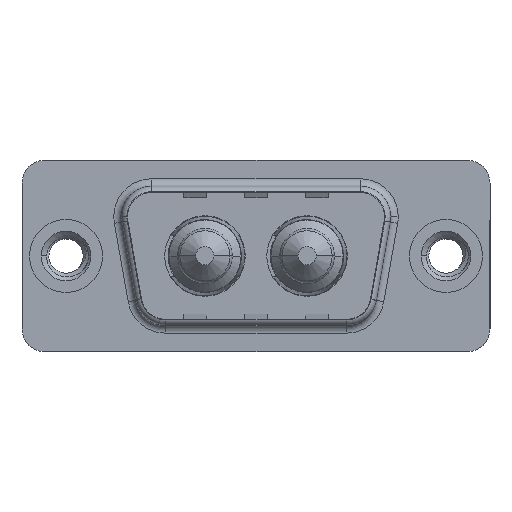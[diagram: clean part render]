
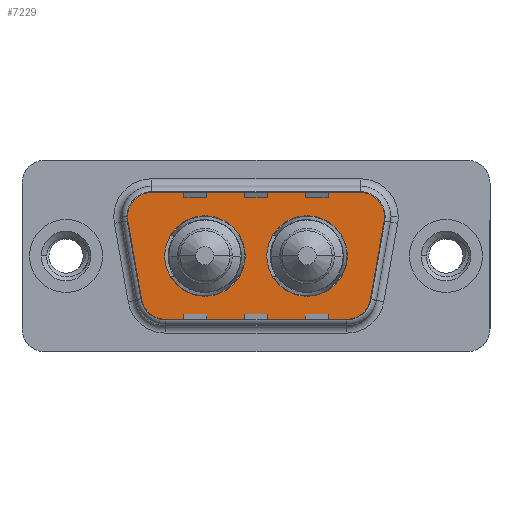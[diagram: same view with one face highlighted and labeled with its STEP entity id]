
A CAD part, top view. The second image highlights one B-rep face of the part: STEP entity #7229.
In plain terms, the highlighted planar face has unit normal (0, 0, 1).
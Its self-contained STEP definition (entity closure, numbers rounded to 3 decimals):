
#38 = VECTOR ( 'NONE', #4921, 1000. ) ;
#371 = CIRCLE ( 'NONE', #11608, 2.65 ) ;
#420 = DIRECTION ( 'NONE',  ( 0.174, -0.985, 0. ) ) ;
#428 = CARTESIAN_POINT ( 'NONE',  ( 19.564, 2.9, 0. ) ) ;
#515 = CIRCLE ( 'NONE', #10790, 2. ) ;
#672 = LINE ( 'NONE', #2986, #10633 ) ;
#941 = CARTESIAN_POINT ( 'NONE',  ( 18.51, 0., 0. ) ) ;
#1047 = DIRECTION ( 'NONE',  ( 0., 0., 1. ) ) ;
#1090 = VERTEX_POINT ( 'NONE', #8661 ) ;
#1092 = AXIS2_PLACEMENT_3D ( 'NONE', #3979, #5673, #10266 ) ;
#1099 = DIRECTION ( 'NONE',  ( -1., 0., 0. ) ) ;
#1525 = VERTEX_POINT ( 'NONE', #3818 ) ;
#1540 = VERTEX_POINT ( 'NONE', #10350 ) ;
#1951 = VERTEX_POINT ( 'NONE', #10084 ) ;
#2005 = CIRCLE ( 'NONE', #5672, 2.65 ) ;
#2106 = DIRECTION ( 'NONE',  ( 1., 0., 0. ) ) ;
#2252 = ORIENTED_EDGE ( 'NONE', *, *, #3138, .T. ) ;
#2335 = EDGE_CURVE ( 'NONE', #10232, #10680, #515, .T. ) ;
#2397 = DIRECTION ( 'NONE',  ( -1., 0., 0. ) ) ;
#2450 = CARTESIAN_POINT ( 'NONE',  ( 18.541, -2.9, 0. ) ) ;
#2498 = ORIENTED_EDGE ( 'NONE', *, *, #2335, .T. ) ;
#2545 = LINE ( 'NONE', #12049, #38 ) ;
#2569 = DIRECTION ( 'NONE',  ( 0., 0., 1. ) ) ;
#2676 = DIRECTION ( 'NONE',  ( 0., 0., 1. ) ) ;
#2828 = ORIENTED_EDGE ( 'NONE', *, *, #12010, .T. ) ;
#2935 = AXIS2_PLACEMENT_3D ( 'NONE', #4379, #2569, #2397 ) ;
#2966 = EDGE_CURVE ( 'NONE', #4654, #9092, #6804, .T. ) ;
#2982 = CARTESIAN_POINT ( 'NONE',  ( 6.459, -4.9, 0. ) ) ;
#2986 = CARTESIAN_POINT ( 'NONE',  ( 5.436, 4.9, 0. ) ) ;
#3026 = LINE ( 'NONE', #6037, #7998 ) ;
#3073 = EDGE_CURVE ( 'NONE', #3878, #1540, #5661, .T. ) ;
#3138 = EDGE_CURVE ( 'NONE', #9092, #10232, #2545, .T. ) ;
#3209 = EDGE_CURVE ( 'NONE', #1951, #8520, #6948, .T. ) ;
#3243 = DIRECTION ( 'NONE',  ( 1., 0., 0. ) ) ;
#3254 = CARTESIAN_POINT ( 'NONE',  ( 18.541, -4.9, 0. ) ) ;
#3329 = CARTESIAN_POINT ( 'NONE',  ( 15.86, 0., 0. ) ) ;
#3336 = DIRECTION ( 'NONE',  ( 1., 0., 0. ) ) ;
#3339 = CARTESIAN_POINT ( 'NONE',  ( 6.459, -2.9, 0. ) ) ;
#3362 = FACE_BOUND ( 'NONE', #8753, .T. ) ;
#3375 = DIRECTION ( 'NONE',  ( 0., 0., 1. ) ) ;
#3466 = DIRECTION ( 'NONE',  ( 0., 0., 1. ) ) ;
#3469 = DIRECTION ( 'NONE',  ( -1., 0., 0. ) ) ;
#3543 = EDGE_CURVE ( 'NONE', #11735, #9312, #10890, .T. ) ;
#3632 = PLANE ( 'NONE',  #6973 ) ;
#3774 = ORIENTED_EDGE ( 'NONE', *, *, #3543, .T. ) ;
#3778 = LINE ( 'NONE', #2982, #6375 ) ;
#3818 = CARTESIAN_POINT ( 'NONE',  ( 19.564, 4.9, 0. ) ) ;
#3878 = VERTEX_POINT ( 'NONE', #7794 ) ;
#3979 = CARTESIAN_POINT ( 'NONE',  ( 5.436, 2.9, 0. ) ) ;
#4060 = CARTESIAN_POINT ( 'NONE',  ( 18.541, -2.9, 0. ) ) ;
#4292 = DIRECTION ( 'NONE',  ( 1., 0., 0. ) ) ;
#4330 = CARTESIAN_POINT ( 'NONE',  ( 3.466, 2.553, 0. ) ) ;
#4379 = CARTESIAN_POINT ( 'NONE',  ( 19.564, 2.9, 0. ) ) ;
#4527 = DIRECTION ( 'NONE',  ( 1., 0., 0. ) ) ;
#4654 = VERTEX_POINT ( 'NONE', #3254 ) ;
#4668 = EDGE_CURVE ( 'NONE', #10680, #1525, #9964, .T. ) ;
#4853 = CARTESIAN_POINT ( 'NONE',  ( 21.564, 2.9, 0. ) ) ;
#4889 = ORIENTED_EDGE ( 'NONE', *, *, #2966, .T. ) ;
#4921 = DIRECTION ( 'NONE',  ( 0.174, 0.985, 0. ) ) ;
#5059 = DIRECTION ( 'NONE',  ( 1., 0., 0. ) ) ;
#5645 = CARTESIAN_POINT ( 'NONE',  ( 9.14, 0., 0. ) ) ;
#5661 = CIRCLE ( 'NONE', #10077, 2.65 ) ;
#5672 = AXIS2_PLACEMENT_3D ( 'NONE', #3329, #9845, #4292 ) ;
#5673 = DIRECTION ( 'NONE',  ( 0., 0., 1. ) ) ;
#5729 = AXIS2_PLACEMENT_3D ( 'NONE', #2450, #1047, #5059 ) ;
#6037 = CARTESIAN_POINT ( 'NONE',  ( 3.466, 2.553, 0. ) ) ;
#6146 = FACE_BOUND ( 'NONE', #10421, .T. ) ;
#6184 = EDGE_CURVE ( 'NONE', #1090, #7620, #6902, .T. ) ;
#6320 = DIRECTION ( 'NONE',  ( 0., 0., 1. ) ) ;
#6331 = CARTESIAN_POINT ( 'NONE',  ( 15.86, 0., 0. ) ) ;
#6375 = VECTOR ( 'NONE', #2106, 1000. ) ;
#6474 = CARTESIAN_POINT ( 'NONE',  ( 20.511, -3.247, 0. ) ) ;
#6541 = DIRECTION ( 'NONE',  ( 1., 0., 0. ) ) ;
#6571 = ORIENTED_EDGE ( 'NONE', *, *, #11302, .T. ) ;
#6627 = ORIENTED_EDGE ( 'NONE', *, *, #12099, .F. ) ;
#6636 = CARTESIAN_POINT ( 'NONE',  ( 6.459, -4.9, 0. ) ) ;
#6804 = CIRCLE ( 'NONE', #5729, 2. ) ;
#6902 = CIRCLE ( 'NONE', #10576, 2.65 ) ;
#6937 = ORIENTED_EDGE ( 'NONE', *, *, #4668, .T. ) ;
#6948 = CIRCLE ( 'NONE', #1092, 2. ) ;
#6973 = AXIS2_PLACEMENT_3D ( 'NONE', #4060, #3466, #3336 ) ;
#7066 = ORIENTED_EDGE ( 'NONE', *, *, #3209, .T. ) ;
#7119 = AXIS2_PLACEMENT_3D ( 'NONE', #3339, #3375, #3469 ) ;
#7229 = ADVANCED_FACE ( 'NONE', ( #3362, #6146, #10540 ), #3632, .T. ) ;
#7620 = VERTEX_POINT ( 'NONE', #941 ) ;
#7794 = CARTESIAN_POINT ( 'NONE',  ( 6.49, 0., 0. ) ) ;
#7911 = DIRECTION ( 'NONE',  ( 0., 0., 1. ) ) ;
#7998 = VECTOR ( 'NONE', #420, 1000. ) ;
#8305 = ORIENTED_EDGE ( 'NONE', *, *, #6184, .F. ) ;
#8520 = VERTEX_POINT ( 'NONE', #4330 ) ;
#8661 = CARTESIAN_POINT ( 'NONE',  ( 13.21, 0., 0. ) ) ;
#8753 = EDGE_LOOP ( 'NONE', ( #6627, #8305 ) ) ;
#8926 = CARTESIAN_POINT ( 'NONE',  ( 21.534, 2.553, 0. ) ) ;
#9030 = ORIENTED_EDGE ( 'NONE', *, *, #3073, .F. ) ;
#9092 = VERTEX_POINT ( 'NONE', #6474 ) ;
#9312 = VERTEX_POINT ( 'NONE', #6636 ) ;
#9543 = EDGE_CURVE ( 'NONE', #8520, #11735, #3026, .T. ) ;
#9609 = ORIENTED_EDGE ( 'NONE', *, *, #11044, .F. ) ;
#9845 = DIRECTION ( 'NONE',  ( 0., 0., 1. ) ) ;
#9964 = CIRCLE ( 'NONE', #2935, 2. ) ;
#10077 = AXIS2_PLACEMENT_3D ( 'NONE', #11256, #2676, #3243 ) ;
#10084 = CARTESIAN_POINT ( 'NONE',  ( 5.436, 4.9, 0. ) ) ;
#10232 = VERTEX_POINT ( 'NONE', #8926 ) ;
#10266 = DIRECTION ( 'NONE',  ( 1., 0., 0. ) ) ;
#10350 = CARTESIAN_POINT ( 'NONE',  ( 11.79, 0., 0. ) ) ;
#10421 = EDGE_LOOP ( 'NONE', ( #9609, #9030 ) ) ;
#10540 = FACE_OUTER_BOUND ( 'NONE', #11295, .T. ) ;
#10576 = AXIS2_PLACEMENT_3D ( 'NONE', #6331, #6320, #4527 ) ;
#10633 = VECTOR ( 'NONE', #11440, 1000. ) ;
#10680 = VERTEX_POINT ( 'NONE', #4853 ) ;
#10790 = AXIS2_PLACEMENT_3D ( 'NONE', #428, #7911, #1099 ) ;
#10890 = CIRCLE ( 'NONE', #7119, 2. ) ;
#11044 = EDGE_CURVE ( 'NONE', #1540, #3878, #371, .T. ) ;
#11256 = CARTESIAN_POINT ( 'NONE',  ( 9.14, 0., 0. ) ) ;
#11295 = EDGE_LOOP ( 'NONE', ( #4889, #2252, #2498, #6937, #2828, #7066, #11606, #3774, #6571 ) ) ;
#11302 = EDGE_CURVE ( 'NONE', #9312, #4654, #3778, .T. ) ;
#11440 = DIRECTION ( 'NONE',  ( -1., 0., 0. ) ) ;
#11606 = ORIENTED_EDGE ( 'NONE', *, *, #9543, .T. ) ;
#11608 = AXIS2_PLACEMENT_3D ( 'NONE', #5645, #12166, #6541 ) ;
#11735 = VERTEX_POINT ( 'NONE', #11980 ) ;
#11980 = CARTESIAN_POINT ( 'NONE',  ( 4.489, -3.247, 0. ) ) ;
#12010 = EDGE_CURVE ( 'NONE', #1525, #1951, #672, .T. ) ;
#12049 = CARTESIAN_POINT ( 'NONE',  ( 21.534, 2.553, 0. ) ) ;
#12099 = EDGE_CURVE ( 'NONE', #7620, #1090, #2005, .T. ) ;
#12166 = DIRECTION ( 'NONE',  ( 0., 0., 1. ) ) ;
